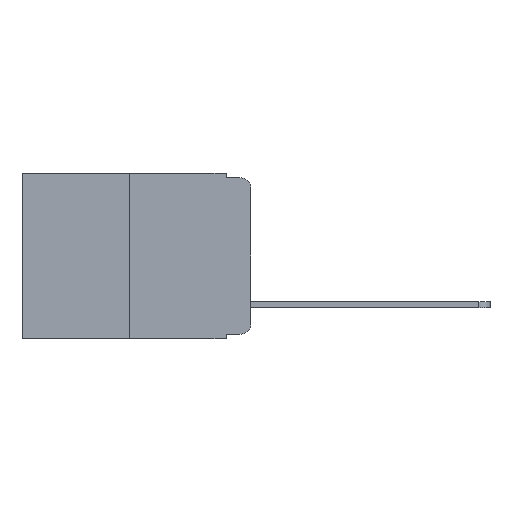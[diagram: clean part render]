
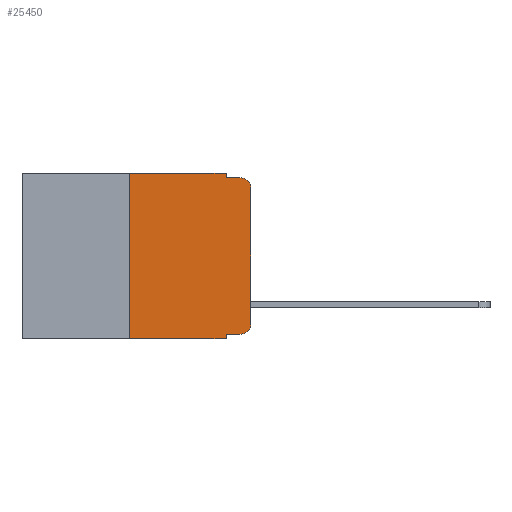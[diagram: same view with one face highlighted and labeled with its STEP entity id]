
A CAD part, left-side view. The second image highlights one B-rep face of the part: STEP entity #25450.
In plain terms, the highlighted planar face has unit normal (-1, 0, 0).
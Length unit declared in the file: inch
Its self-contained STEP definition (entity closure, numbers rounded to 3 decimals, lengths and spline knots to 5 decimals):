
#507 = EDGE_CURVE ( 'NONE', #2347, #14650, #23953, .T. ) ;
#770 = VERTEX_POINT ( 'NONE', #9967 ) ;
#949 = AXIS2_PLACEMENT_3D ( 'NONE', #12541, #26020, #14505 ) ;
#1319 = VECTOR ( 'NONE', #7924, 39.37008 ) ;
#1615 = CARTESIAN_POINT ( 'NONE',  ( 0., 0., -0.313 ) ) ;
#2045 = CARTESIAN_POINT ( 'NONE',  ( 0., 0.051, -0.01 ) ) ;
#2347 = VERTEX_POINT ( 'NONE', #1615 ) ;
#2392 = CARTESIAN_POINT ( 'NONE',  ( 0., 0.051, -0.333 ) ) ;
#2541 = DIRECTION ( 'NONE',  ( 0., -1., 0. ) ) ;
#4397 = LINE ( 'NONE', #10010, #24721 ) ;
#4421 = ORIENTED_EDGE ( 'NONE', *, *, #14062, .T. ) ;
#4611 = EDGE_CURVE ( 'NONE', #7914, #2347, #15770, .T. ) ;
#5040 = VERTEX_POINT ( 'NONE', #20160 ) ;
#5084 = CARTESIAN_POINT ( 'NONE',  ( 0., 0.25, 0. ) ) ;
#5139 = DIRECTION ( 'NONE',  ( -1., 0., 0. ) ) ;
#5499 = EDGE_CURVE ( 'NONE', #5849, #25120, #13355, .T. ) ;
#5556 = LINE ( 'NONE', #2045, #15549 ) ;
#5849 = VERTEX_POINT ( 'NONE', #2392 ) ;
#6066 = EDGE_LOOP ( 'NONE', ( #21893, #15272, #22233, #18340, #23183, #17754, #10176, #25026, #4421, #10745 ) ) ;
#6152 = LINE ( 'NONE', #24071, #16122 ) ;
#6336 = CARTESIAN_POINT ( 'NONE',  ( 0., 0., -0.03 ) ) ;
#6779 = DIRECTION ( 'NONE',  ( 0., 0., 1. ) ) ;
#6845 = EDGE_CURVE ( 'NONE', #24151, #17116, #4397, .T. ) ;
#7018 = CARTESIAN_POINT ( 'NONE',  ( 0., 0.02, -0.333 ) ) ;
#7161 = LINE ( 'NONE', #13774, #1319 ) ;
#7780 = DIRECTION ( 'NONE',  ( 0., 0., -1. ) ) ;
#7914 = VERTEX_POINT ( 'NONE', #7018 ) ;
#7924 = DIRECTION ( 'NONE',  ( 0., -1., 0. ) ) ;
#9729 = EDGE_CURVE ( 'NONE', #17116, #16298, #7161, .T. ) ;
#9967 = CARTESIAN_POINT ( 'NONE',  ( 0., 0.02, -0.01 ) ) ;
#10010 = CARTESIAN_POINT ( 'NONE',  ( 0., 0.25, 0. ) ) ;
#10176 = ORIENTED_EDGE ( 'NONE', *, *, #10463, .T. ) ;
#10289 = LINE ( 'NONE', #21427, #25154 ) ;
#10463 = EDGE_CURVE ( 'NONE', #24151, #25120, #6152, .T. ) ;
#10745 = ORIENTED_EDGE ( 'NONE', *, *, #4611, .T. ) ;
#11380 = LINE ( 'NONE', #18704, #20511 ) ;
#11773 = DIRECTION ( 'NONE',  ( 0., 0., -1. ) ) ;
#12541 = CARTESIAN_POINT ( 'NONE',  ( 0., 0.02, -0.03 ) ) ;
#12585 = CIRCLE ( 'NONE', #949, 0.02 ) ;
#12591 = CARTESIAN_POINT ( 'NONE',  ( 0., 0.473, 0. ) ) ;
#12653 = CARTESIAN_POINT ( 'NONE',  ( 0., 0.25, -0.343 ) ) ;
#12747 = VECTOR ( 'NONE', #7780, 39.37008 ) ;
#12792 = CARTESIAN_POINT ( 'NONE',  ( 0., 0., 0. ) ) ;
#13355 = LINE ( 'NONE', #23410, #12747 ) ;
#13774 = CARTESIAN_POINT ( 'NONE',  ( 0., 0.473, 0. ) ) ;
#14062 = EDGE_CURVE ( 'NONE', #5849, #7914, #11380, .T. ) ;
#14505 = DIRECTION ( 'NONE',  ( 0., 0., -1. ) ) ;
#14553 = DIRECTION ( 'NONE',  ( 0., 0., -1. ) ) ;
#14650 = VERTEX_POINT ( 'NONE', #6336 ) ;
#15272 = ORIENTED_EDGE ( 'NONE', *, *, #22785, .T. ) ;
#15549 = VECTOR ( 'NONE', #24105, 39.37008 ) ;
#15770 = CIRCLE ( 'NONE', #25705, 0.02 ) ;
#16122 = VECTOR ( 'NONE', #26010, 39.37008 ) ;
#16298 = VERTEX_POINT ( 'NONE', #24319 ) ;
#16404 = PLANE ( 'NONE',  #16709 ) ;
#16709 = AXIS2_PLACEMENT_3D ( 'NONE', #12591, #26062, #14553 ) ;
#17027 = CARTESIAN_POINT ( 'NONE',  ( 0., 0.02, -0.313 ) ) ;
#17116 = VERTEX_POINT ( 'NONE', #5084 ) ;
#17593 = EDGE_CURVE ( 'NONE', #5040, #770, #5556, .T. ) ;
#17754 = ORIENTED_EDGE ( 'NONE', *, *, #6845, .F. ) ;
#18340 = ORIENTED_EDGE ( 'NONE', *, *, #24528, .F. ) ;
#18704 = CARTESIAN_POINT ( 'NONE',  ( 0., 0.051, -0.333 ) ) ;
#18830 = VECTOR ( 'NONE', #6779, 39.37008 ) ;
#18971 = DIRECTION ( 'NONE',  ( 0., 0., -1. ) ) ;
#19276 = CARTESIAN_POINT ( 'NONE',  ( 0., 0.051, -0.343 ) ) ;
#20160 = CARTESIAN_POINT ( 'NONE',  ( 0., 0.051, -0.01 ) ) ;
#20511 = VECTOR ( 'NONE', #2541, 39.37008 ) ;
#21427 = CARTESIAN_POINT ( 'NONE',  ( 0., 0.051, 0. ) ) ;
#21893 = ORIENTED_EDGE ( 'NONE', *, *, #507, .T. ) ;
#22233 = ORIENTED_EDGE ( 'NONE', *, *, #17593, .F. ) ;
#22724 = FACE_OUTER_BOUND ( 'NONE', #6066, .T. ) ;
#22785 = EDGE_CURVE ( 'NONE', #14650, #770, #12585, .T. ) ;
#23183 = ORIENTED_EDGE ( 'NONE', *, *, #9729, .F. ) ;
#23410 = CARTESIAN_POINT ( 'NONE',  ( 0., 0.051, 0. ) ) ;
#23953 = LINE ( 'NONE', #12792, #18830 ) ;
#24071 = CARTESIAN_POINT ( 'NONE',  ( 0., 0.473, -0.343 ) ) ;
#24105 = DIRECTION ( 'NONE',  ( 0., -1., 0. ) ) ;
#24151 = VERTEX_POINT ( 'NONE', #12653 ) ;
#24319 = CARTESIAN_POINT ( 'NONE',  ( 0., 0.051, 0. ) ) ;
#24528 = EDGE_CURVE ( 'NONE', #16298, #5040, #10289, .T. ) ;
#24721 = VECTOR ( 'NONE', #25512, 39.37008 ) ;
#25026 = ORIENTED_EDGE ( 'NONE', *, *, #5499, .F. ) ;
#25120 = VERTEX_POINT ( 'NONE', #19276 ) ;
#25154 = VECTOR ( 'NONE', #11773, 39.37008 ) ;
#25450 = ADVANCED_FACE ( 'NONE', ( #22724 ), #16404, .F. ) ;
#25512 = DIRECTION ( 'NONE',  ( 0., 0., 1. ) ) ;
#25705 = AXIS2_PLACEMENT_3D ( 'NONE', #17027, #5139, #18971 ) ;
#26010 = DIRECTION ( 'NONE',  ( 0., -1., 0. ) ) ;
#26020 = DIRECTION ( 'NONE',  ( -1., 0., 0. ) ) ;
#26062 = DIRECTION ( 'NONE',  ( 1., 0., 0. ) ) ;
